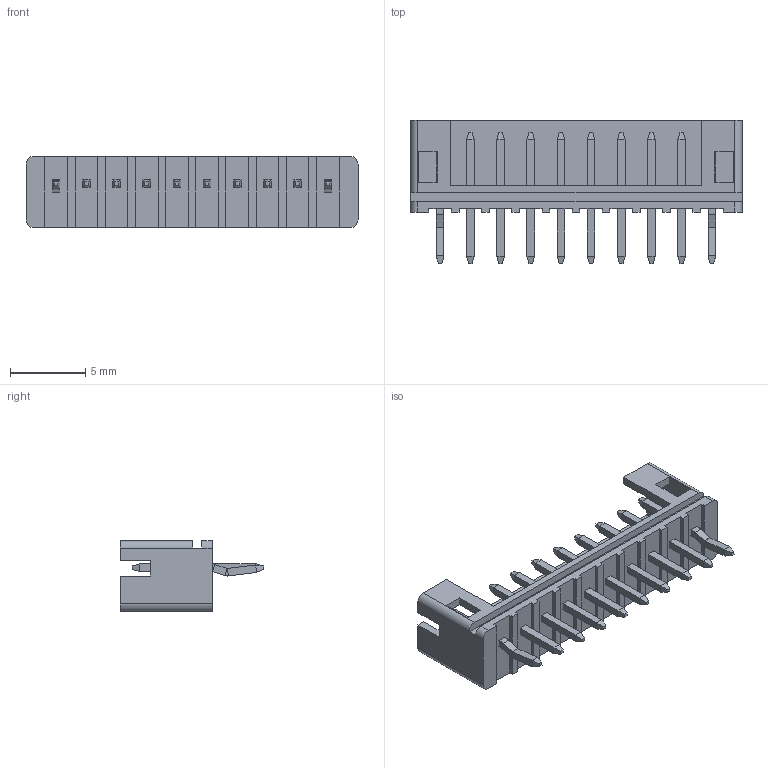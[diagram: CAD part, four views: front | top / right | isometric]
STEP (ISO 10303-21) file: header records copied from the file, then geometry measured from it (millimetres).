
FILE_DESCRIPTION (( 'STEP AP203' ), '1' );
FILE_NAME ('140-510-415-001.STEP', '2020-03-31T19:24:03', ( '' ), ( '' ), 'SwSTEP 2.0', 'SolidWorks 2016', '' );
FILE_SCHEMA (( 'CONFIG_CONTROL_DESIGN' ));
Length unit declared in the file: millimetre
Products named in the file (4): V Contact_Str; 140-510-415-001; V Housing_510; V Contact_Kink
Assembly tree (11 placements, depth 2):
  140-510-415-001
    V Housing_510
    V Contact_Kink  x2
    V Contact_Str  x8
Bounding box: 22 x 9.51 x 4.7 mm (x, y, z)
Volume: 232.4 mm3; surface area: 850 mm2
Topology: 11 solids, 11 shells, 290 faces, 706 edges, 436 vertices
Faces by surface type: plane 272, cylinder 16, bspline 2
Entity records: 5795 total; most frequent: CARTESIAN_POINT 947, ORIENTED_EDGE 894, DIRECTION 823, EDGE_CURVE 447, LINE 423, VECTOR 423, VERTEX_POINT 288, AXIS2_PLACEMENT_3D 200
